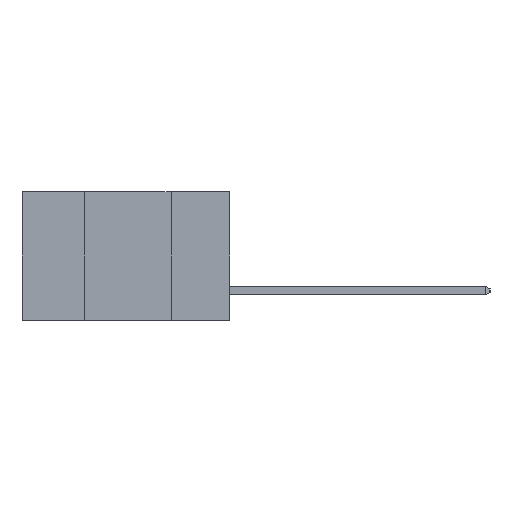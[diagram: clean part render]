
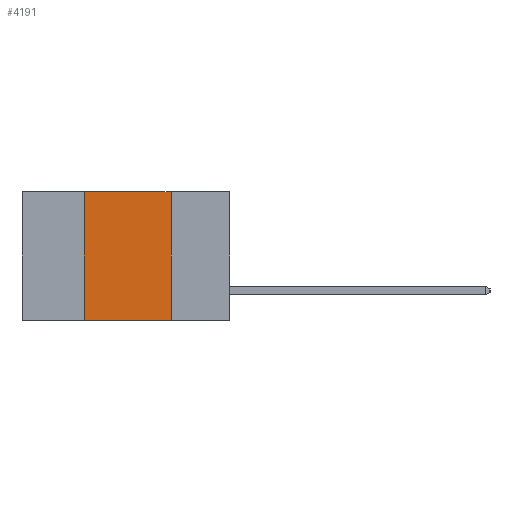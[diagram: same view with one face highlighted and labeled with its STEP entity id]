
A CAD part, left-side view. The second image highlights one B-rep face of the part: STEP entity #4191.
In plain terms, the highlighted planar face has unit normal (-1, 0, 0).
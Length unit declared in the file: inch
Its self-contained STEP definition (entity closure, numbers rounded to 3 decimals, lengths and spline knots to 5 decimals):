
#899 = AXIS2_PLACEMENT_3D ( 'NONE', #12697, #11952, #7901 ) ;
#1243 = VECTOR ( 'NONE', #7860, 39.37008 ) ;
#1606 = FACE_OUTER_BOUND ( 'NONE', #12563, .T. ) ;
#1784 = LINE ( 'NONE', #10431, #10757 ) ;
#2286 = DIRECTION ( 'NONE',  ( 0., -1., 0. ) ) ;
#2572 = LINE ( 'NONE', #7721, #5414 ) ;
#2761 = VERTEX_POINT ( 'NONE', #8611 ) ;
#3063 = VECTOR ( 'NONE', #11877, 39.37008 ) ;
#3608 = VERTEX_POINT ( 'NONE', #6227 ) ;
#4191 = ADVANCED_FACE ( 'NONE', ( #1606 ), #12797, .F. ) ;
#5414 = VECTOR ( 'NONE', #11079, 39.37008 ) ;
#5502 = EDGE_CURVE ( 'NONE', #13548, #3608, #1784, .T. ) ;
#6227 = CARTESIAN_POINT ( 'NONE',  ( 0., 0.17, 0. ) ) ;
#6265 = CARTESIAN_POINT ( 'NONE',  ( 0., 0.17, 0. ) ) ;
#6692 = CARTESIAN_POINT ( 'NONE',  ( 0., 0.42, 0. ) ) ;
#6913 = CARTESIAN_POINT ( 'NONE',  ( 0., 0.42, -0.37 ) ) ;
#7229 = LINE ( 'NONE', #13335, #1243 ) ;
#7721 = CARTESIAN_POINT ( 'NONE',  ( 0., 0.6, -0.37 ) ) ;
#7860 = DIRECTION ( 'NONE',  ( 0., 0., 1. ) ) ;
#7901 = DIRECTION ( 'NONE',  ( 0., 0., -1. ) ) ;
#8366 = EDGE_CURVE ( 'NONE', #9776, #2761, #2572, .T. ) ;
#8611 = CARTESIAN_POINT ( 'NONE',  ( 0., 0.17, -0.37 ) ) ;
#9124 = EDGE_CURVE ( 'NONE', #9776, #13548, #7229, .T. ) ;
#9776 = VERTEX_POINT ( 'NONE', #6913 ) ;
#10431 = CARTESIAN_POINT ( 'NONE',  ( 0., 0.6, 0. ) ) ;
#10578 = EDGE_CURVE ( 'NONE', #3608, #2761, #14757, .T. ) ;
#10757 = VECTOR ( 'NONE', #2286, 39.37008 ) ;
#10958 = ORIENTED_EDGE ( 'NONE', *, *, #9124, .F. ) ;
#11079 = DIRECTION ( 'NONE',  ( 0., -1., 0. ) ) ;
#11137 = ORIENTED_EDGE ( 'NONE', *, *, #5502, .F. ) ;
#11254 = ORIENTED_EDGE ( 'NONE', *, *, #10578, .F. ) ;
#11877 = DIRECTION ( 'NONE',  ( 0., 0., -1. ) ) ;
#11952 = DIRECTION ( 'NONE',  ( 1., 0., 0. ) ) ;
#12563 = EDGE_LOOP ( 'NONE', ( #11254, #11137, #10958, #14124 ) ) ;
#12697 = CARTESIAN_POINT ( 'NONE',  ( 0., 0.6, 0. ) ) ;
#12797 = PLANE ( 'NONE',  #899 ) ;
#13335 = CARTESIAN_POINT ( 'NONE',  ( 0., 0.42, 0. ) ) ;
#13548 = VERTEX_POINT ( 'NONE', #6692 ) ;
#14124 = ORIENTED_EDGE ( 'NONE', *, *, #8366, .T. ) ;
#14757 = LINE ( 'NONE', #6265, #3063 ) ;
